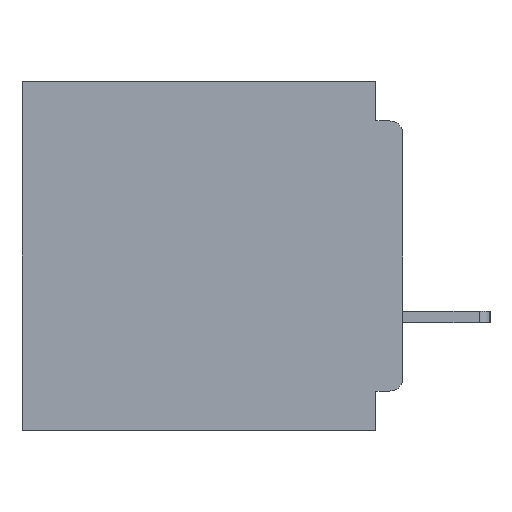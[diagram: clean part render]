
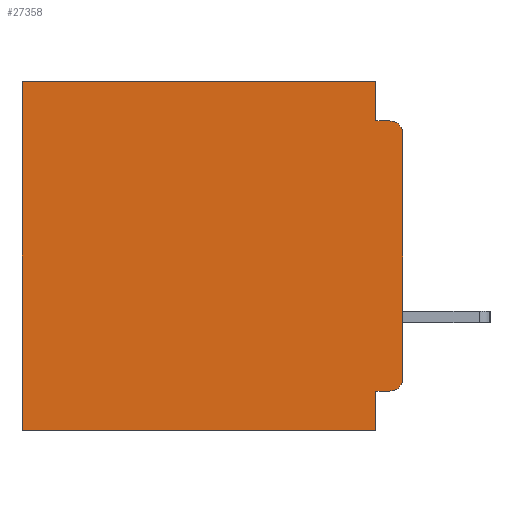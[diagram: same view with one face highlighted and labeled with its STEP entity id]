
A CAD part, left-side view. The second image highlights one B-rep face of the part: STEP entity #27358.
In plain terms, the highlighted planar face has unit normal (-1, 0, 0).
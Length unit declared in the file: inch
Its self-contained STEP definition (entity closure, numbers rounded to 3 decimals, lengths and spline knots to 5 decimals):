
#52 = VERTEX_POINT ( 'NONE', #33256 ) ;
#308 = CARTESIAN_POINT ( 'NONE',  ( 0.3, 0., -0.355 ) ) ;
#2356 = VECTOR ( 'NONE', #26888, 39.37008 ) ;
#2629 = DIRECTION ( 'NONE',  ( 0., 0., -1. ) ) ;
#2726 = EDGE_CURVE ( 'NONE', #4756, #24310, #28023, .T. ) ;
#3534 = DIRECTION ( 'NONE',  ( 0., 0., -1. ) ) ;
#3671 = ORIENTED_EDGE ( 'NONE', *, *, #31392, .F. ) ;
#4695 = VERTEX_POINT ( 'NONE', #26837 ) ;
#4756 = VERTEX_POINT ( 'NONE', #25993 ) ;
#6631 = ORIENTED_EDGE ( 'NONE', *, *, #22850, .F. ) ;
#7245 = VECTOR ( 'NONE', #19320, 39.37008 ) ;
#7781 = VECTOR ( 'NONE', #13903, 39.37008 ) ;
#7968 = VERTEX_POINT ( 'NONE', #13417 ) ;
#8055 = LINE ( 'NONE', #11039, #39584 ) ;
#8322 = CARTESIAN_POINT ( 'NONE',  ( 0.3, 0.031, -0.4 ) ) ;
#8568 = ORIENTED_EDGE ( 'NONE', *, *, #26499, .T. ) ;
#8722 = ORIENTED_EDGE ( 'NONE', *, *, #11079, .T. ) ;
#8773 = CARTESIAN_POINT ( 'NONE',  ( 0.3, 0., -0.045 ) ) ;
#8780 = VECTOR ( 'NONE', #15908, 39.37008 ) ;
#10281 = VERTEX_POINT ( 'NONE', #26291 ) ;
#10683 = VECTOR ( 'NONE', #30254, 39.37008 ) ;
#11039 = CARTESIAN_POINT ( 'NONE',  ( 0.3, 0., 0. ) ) ;
#11079 = EDGE_CURVE ( 'NONE', #4756, #52, #32717, .T. ) ;
#11869 = AXIS2_PLACEMENT_3D ( 'NONE', #33005, #14784, #36095 ) ;
#12016 = EDGE_CURVE ( 'NONE', #20618, #52, #24214, .T. ) ;
#13196 = DIRECTION ( 'NONE',  ( 1., 0., 0. ) ) ;
#13417 = CARTESIAN_POINT ( 'NONE',  ( 0.3, 0.031, -0.045 ) ) ;
#13903 = DIRECTION ( 'NONE',  ( 0., 0., -1. ) ) ;
#14784 = DIRECTION ( 'NONE',  ( -1., 0., 0. ) ) ;
#15742 = AXIS2_PLACEMENT_3D ( 'NONE', #19262, #13196, #34537 ) ;
#15908 = DIRECTION ( 'NONE',  ( 0., 1., 0. ) ) ;
#15953 = CARTESIAN_POINT ( 'NONE',  ( 0.3, 0.031, -0.4 ) ) ;
#16808 = FACE_OUTER_BOUND ( 'NONE', #18073, .T. ) ;
#17008 = LINE ( 'NONE', #28107, #8780 ) ;
#18073 = EDGE_LOOP ( 'NONE', ( #24472, #8568, #3671, #6631, #27898, #37787, #30705, #35935, #29842, #8722 ) ) ;
#18435 = CARTESIAN_POINT ( 'NONE',  ( 0.3, 0.031, -0.355 ) ) ;
#18716 = VERTEX_POINT ( 'NONE', #29840 ) ;
#18889 = LINE ( 'NONE', #8773, #10683 ) ;
#19262 = CARTESIAN_POINT ( 'NONE',  ( 0.3, 0., -0.4 ) ) ;
#19320 = DIRECTION ( 'NONE',  ( 0., 0., -1. ) ) ;
#20082 = AXIS2_PLACEMENT_3D ( 'NONE', #39360, #21237, #2629 ) ;
#20618 = VERTEX_POINT ( 'NONE', #26250 ) ;
#21237 = DIRECTION ( 'NONE',  ( -1., 0., 0. ) ) ;
#21557 = EDGE_CURVE ( 'NONE', #24310, #36256, #24753, .T. ) ;
#22136 = EDGE_CURVE ( 'NONE', #36256, #26199, #17008, .T. ) ;
#22850 = EDGE_CURVE ( 'NONE', #18716, #7968, #31728, .T. ) ;
#23308 = DIRECTION ( 'NONE',  ( 0., 1., 0. ) ) ;
#23722 = LINE ( 'NONE', #36558, #29888 ) ;
#24214 = LINE ( 'NONE', #38286, #7781 ) ;
#24310 = VERTEX_POINT ( 'NONE', #18435 ) ;
#24472 = ORIENTED_EDGE ( 'NONE', *, *, #12016, .F. ) ;
#24753 = LINE ( 'NONE', #15953, #38935 ) ;
#25393 = CARTESIAN_POINT ( 'NONE',  ( 0.3, 0.031, 0. ) ) ;
#25993 = CARTESIAN_POINT ( 'NONE',  ( 0.3, 0.015, -0.355 ) ) ;
#26044 = CIRCLE ( 'NONE', #20082, 0.015 ) ;
#26199 = VERTEX_POINT ( 'NONE', #31860 ) ;
#26250 = CARTESIAN_POINT ( 'NONE',  ( 0.3, 0., -0.06 ) ) ;
#26291 = CARTESIAN_POINT ( 'NONE',  ( 0.3, 0.015, -0.045 ) ) ;
#26499 = EDGE_CURVE ( 'NONE', #20618, #10281, #26044, .T. ) ;
#26837 = CARTESIAN_POINT ( 'NONE',  ( 0.3, 0.437, 0. ) ) ;
#26888 = DIRECTION ( 'NONE',  ( 0., 1., 0. ) ) ;
#27358 = ADVANCED_FACE ( 'NONE', ( #16808 ), #28516, .F. ) ;
#27568 = EDGE_CURVE ( 'NONE', #18716, #4695, #8055, .T. ) ;
#27898 = ORIENTED_EDGE ( 'NONE', *, *, #27568, .T. ) ;
#28023 = LINE ( 'NONE', #308, #2356 ) ;
#28107 = CARTESIAN_POINT ( 'NONE',  ( 0.3, 0., -0.4 ) ) ;
#28516 = PLANE ( 'NONE',  #15742 ) ;
#29840 = CARTESIAN_POINT ( 'NONE',  ( 0.3, 0.031, 0. ) ) ;
#29842 = ORIENTED_EDGE ( 'NONE', *, *, #2726, .F. ) ;
#29888 = VECTOR ( 'NONE', #39570, 39.37008 ) ;
#30254 = DIRECTION ( 'NONE',  ( 0., -1., 0. ) ) ;
#30705 = ORIENTED_EDGE ( 'NONE', *, *, #22136, .F. ) ;
#31392 = EDGE_CURVE ( 'NONE', #7968, #10281, #18889, .T. ) ;
#31728 = LINE ( 'NONE', #25393, #7245 ) ;
#31860 = CARTESIAN_POINT ( 'NONE',  ( 0.3, 0.437, -0.4 ) ) ;
#32103 = EDGE_CURVE ( 'NONE', #4695, #26199, #23722, .T. ) ;
#32717 = CIRCLE ( 'NONE', #11869, 0.015 ) ;
#33005 = CARTESIAN_POINT ( 'NONE',  ( 0.3, 0.015, -0.34 ) ) ;
#33256 = CARTESIAN_POINT ( 'NONE',  ( 0.3, 0., -0.34 ) ) ;
#34537 = DIRECTION ( 'NONE',  ( 0., 0., -1. ) ) ;
#35935 = ORIENTED_EDGE ( 'NONE', *, *, #21557, .F. ) ;
#36095 = DIRECTION ( 'NONE',  ( 0., 0., -1. ) ) ;
#36256 = VERTEX_POINT ( 'NONE', #8322 ) ;
#36558 = CARTESIAN_POINT ( 'NONE',  ( 0.3, 0.437, -0.4 ) ) ;
#37787 = ORIENTED_EDGE ( 'NONE', *, *, #32103, .T. ) ;
#38286 = CARTESIAN_POINT ( 'NONE',  ( 0.3, 0., -0.4 ) ) ;
#38935 = VECTOR ( 'NONE', #3534, 39.37008 ) ;
#39360 = CARTESIAN_POINT ( 'NONE',  ( 0.3, 0.015, -0.06 ) ) ;
#39570 = DIRECTION ( 'NONE',  ( 0., 0., -1. ) ) ;
#39584 = VECTOR ( 'NONE', #23308, 39.37008 ) ;
